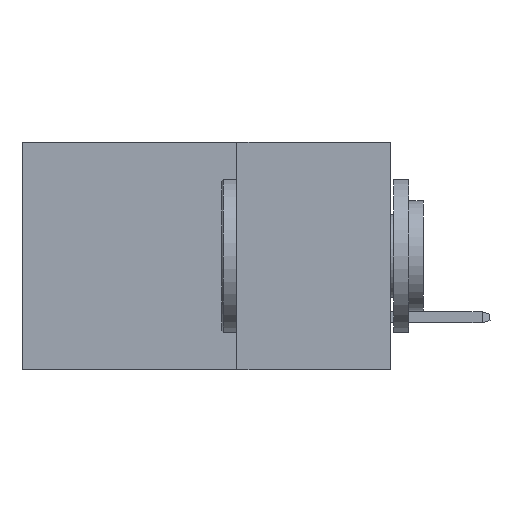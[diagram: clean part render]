
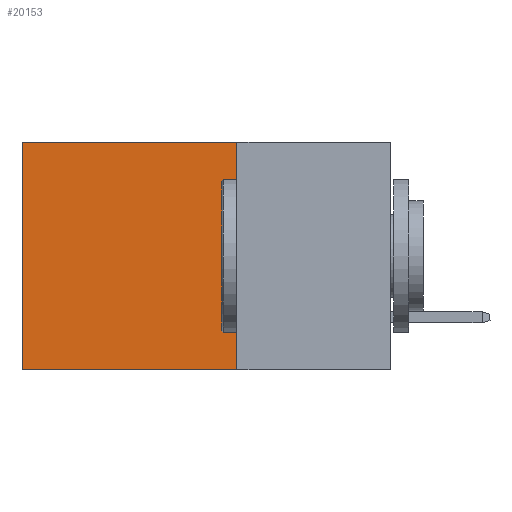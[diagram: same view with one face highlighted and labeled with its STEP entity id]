
A CAD part, left-side view. The second image highlights one B-rep face of the part: STEP entity #20153.
In plain terms, the highlighted planar face has unit normal (-1, 0, 0).
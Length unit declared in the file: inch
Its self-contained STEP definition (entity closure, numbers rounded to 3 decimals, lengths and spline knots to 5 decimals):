
#161 = EDGE_CURVE ( 'NONE', #19182, #6803, #27200, .T. ) ;
#299 = CARTESIAN_POINT ( 'NONE',  ( 0.2875, 0.6, 0. ) ) ;
#902 = CARTESIAN_POINT ( 'NONE',  ( 0.2875, 0.25, -0.37 ) ) ;
#1751 = ORIENTED_EDGE ( 'NONE', *, *, #25322, .T. ) ;
#1910 = DIRECTION ( 'NONE',  ( 0., 1., 0. ) ) ;
#4228 = CARTESIAN_POINT ( 'NONE',  ( 0.2875, 0.6, -0.37 ) ) ;
#4373 = ORIENTED_EDGE ( 'NONE', *, *, #161, .F. ) ;
#4483 = EDGE_CURVE ( 'NONE', #6803, #28067, #18134, .T. ) ;
#5098 = VECTOR ( 'NONE', #11822, 39.37008 ) ;
#6774 = AXIS2_PLACEMENT_3D ( 'NONE', #22707, #25488, #8679 ) ;
#6803 = VERTEX_POINT ( 'NONE', #902 ) ;
#8553 = PLANE ( 'NONE',  #6774 ) ;
#8679 = DIRECTION ( 'NONE',  ( 0., 0., -1. ) ) ;
#9350 = EDGE_CURVE ( 'NONE', #19182, #30683, #28962, .T. ) ;
#10637 = VECTOR ( 'NONE', #1910, 39.37008 ) ;
#11822 = DIRECTION ( 'NONE',  ( 0., 0., -1. ) ) ;
#12306 = VECTOR ( 'NONE', #29183, 39.37008 ) ;
#14332 = ORIENTED_EDGE ( 'NONE', *, *, #9350, .T. ) ;
#14930 = VECTOR ( 'NONE', #15390, 39.37008 ) ;
#15390 = DIRECTION ( 'NONE',  ( 0., 1., 0. ) ) ;
#18134 = LINE ( 'NONE', #24618, #10637 ) ;
#19182 = VERTEX_POINT ( 'NONE', #28953 ) ;
#19609 = EDGE_LOOP ( 'NONE', ( #1751, #35963, #4373, #14332 ) ) ;
#20153 = ADVANCED_FACE ( 'NONE', ( #25306 ), #8553, .F. ) ;
#22707 = CARTESIAN_POINT ( 'NONE',  ( 0.2875, 0.25, 0. ) ) ;
#24618 = CARTESIAN_POINT ( 'NONE',  ( 0.2875, 0.25, -0.37 ) ) ;
#25306 = FACE_OUTER_BOUND ( 'NONE', #19609, .T. ) ;
#25322 = EDGE_CURVE ( 'NONE', #30683, #28067, #35035, .T. ) ;
#25369 = CARTESIAN_POINT ( 'NONE',  ( 0.2875, 0.6, 0. ) ) ;
#25488 = DIRECTION ( 'NONE',  ( 1., 0., 0. ) ) ;
#27200 = LINE ( 'NONE', #29352, #12306 ) ;
#28067 = VERTEX_POINT ( 'NONE', #4228 ) ;
#28953 = CARTESIAN_POINT ( 'NONE',  ( 0.2875, 0.25, 0. ) ) ;
#28962 = LINE ( 'NONE', #34961, #14930 ) ;
#29183 = DIRECTION ( 'NONE',  ( 0., 0., -1. ) ) ;
#29352 = CARTESIAN_POINT ( 'NONE',  ( 0.2875, 0.25, 0. ) ) ;
#30683 = VERTEX_POINT ( 'NONE', #25369 ) ;
#34961 = CARTESIAN_POINT ( 'NONE',  ( 0.2875, 0.25, 0. ) ) ;
#35035 = LINE ( 'NONE', #299, #5098 ) ;
#35963 = ORIENTED_EDGE ( 'NONE', *, *, #4483, .F. ) ;
